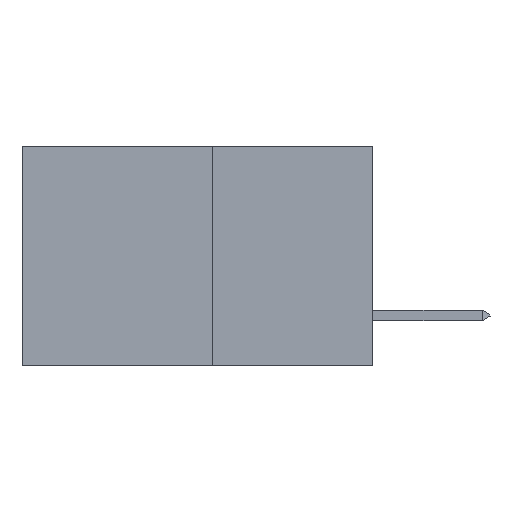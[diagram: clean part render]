
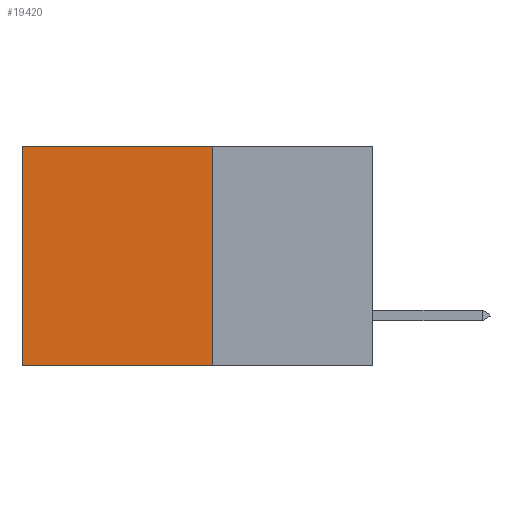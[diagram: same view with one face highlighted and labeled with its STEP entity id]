
A CAD part, left-side view. The second image highlights one B-rep face of the part: STEP entity #19420.
In plain terms, the highlighted planar face has unit normal (-1, 0, 0).
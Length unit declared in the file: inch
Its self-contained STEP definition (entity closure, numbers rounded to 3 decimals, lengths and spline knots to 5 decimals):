
#378 = CARTESIAN_POINT ( 'NONE',  ( 0.277, 0.27, 0. ) ) ;
#1594 = VERTEX_POINT ( 'NONE', #14778 ) ;
#2208 = DIRECTION ( 'NONE',  ( 0., 0., -1. ) ) ;
#2852 = EDGE_CURVE ( 'NONE', #5475, #1594, #21484, .T. ) ;
#2975 = DIRECTION ( 'NONE',  ( 0., 0., -1. ) ) ;
#3354 = LINE ( 'NONE', #12512, #29722 ) ;
#5350 = AXIS2_PLACEMENT_3D ( 'NONE', #18402, #23346, #2975 ) ;
#5475 = VERTEX_POINT ( 'NONE', #6808 ) ;
#6135 = ORIENTED_EDGE ( 'NONE', *, *, #29420, .F. ) ;
#6509 = LINE ( 'NONE', #378, #18605 ) ;
#6808 = CARTESIAN_POINT ( 'NONE',  ( 0.277, 0.27, 0. ) ) ;
#7846 = DIRECTION ( 'NONE',  ( 0., 1., 0. ) ) ;
#8039 = PLANE ( 'NONE',  #5350 ) ;
#10342 = CARTESIAN_POINT ( 'NONE',  ( 0.277, 0.27, -0.37 ) ) ;
#10623 = CARTESIAN_POINT ( 'NONE',  ( 0.277, 0.59, -0.37 ) ) ;
#12512 = CARTESIAN_POINT ( 'NONE',  ( 0.277, 0.59, -0.37 ) ) ;
#12719 = EDGE_CURVE ( 'NONE', #5475, #17897, #6509, .T. ) ;
#14759 = VECTOR ( 'NONE', #32435, 39.37008 ) ;
#14778 = CARTESIAN_POINT ( 'NONE',  ( 0.277, 0.27, -0.37 ) ) ;
#15477 = VERTEX_POINT ( 'NONE', #10623 ) ;
#17897 = VERTEX_POINT ( 'NONE', #32376 ) ;
#18402 = CARTESIAN_POINT ( 'NONE',  ( 0.277, 0.27, -0.37 ) ) ;
#18605 = VECTOR ( 'NONE', #22967, 39.37008 ) ;
#19033 = ORIENTED_EDGE ( 'NONE', *, *, #26173, .T. ) ;
#19036 = CARTESIAN_POINT ( 'NONE',  ( 0.277, 0.27, -0.37 ) ) ;
#19420 = ADVANCED_FACE ( 'NONE', ( #21358 ), #8039, .F. ) ;
#20532 = VECTOR ( 'NONE', #7846, 39.37008 ) ;
#21358 = FACE_OUTER_BOUND ( 'NONE', #31109, .T. ) ;
#21361 = ORIENTED_EDGE ( 'NONE', *, *, #2852, .F. ) ;
#21484 = LINE ( 'NONE', #19036, #14759 ) ;
#22967 = DIRECTION ( 'NONE',  ( 0., 1., 0. ) ) ;
#23346 = DIRECTION ( 'NONE',  ( 1., 0., 0. ) ) ;
#26173 = EDGE_CURVE ( 'NONE', #17897, #15477, #3354, .T. ) ;
#26940 = ORIENTED_EDGE ( 'NONE', *, *, #12719, .T. ) ;
#28042 = LINE ( 'NONE', #10342, #20532 ) ;
#29420 = EDGE_CURVE ( 'NONE', #1594, #15477, #28042, .T. ) ;
#29722 = VECTOR ( 'NONE', #2208, 39.37008 ) ;
#31109 = EDGE_LOOP ( 'NONE', ( #19033, #6135, #21361, #26940 ) ) ;
#32376 = CARTESIAN_POINT ( 'NONE',  ( 0.277, 0.59, 0. ) ) ;
#32435 = DIRECTION ( 'NONE',  ( 0., 0., -1. ) ) ;
